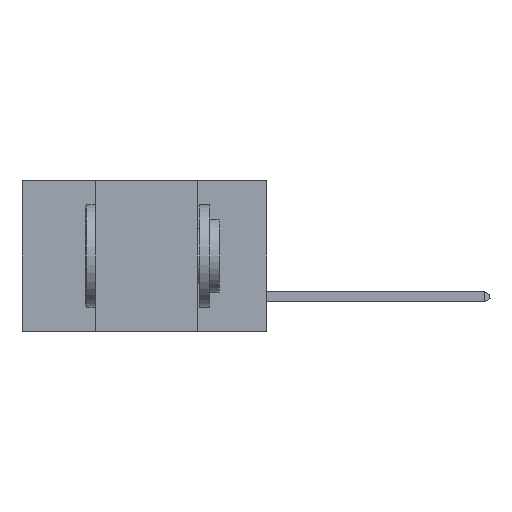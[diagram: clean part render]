
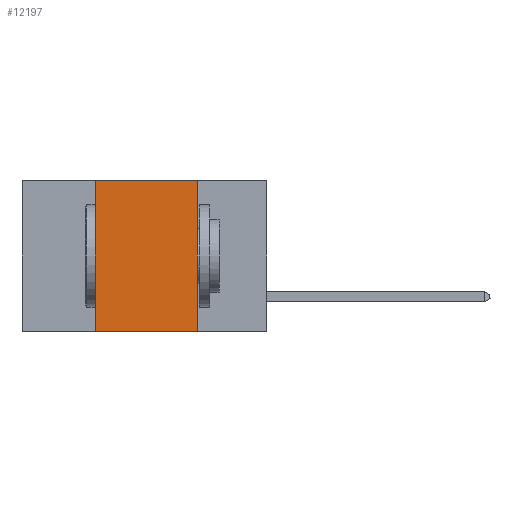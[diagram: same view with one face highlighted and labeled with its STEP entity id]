
A CAD part, left-side view. The second image highlights one B-rep face of the part: STEP entity #12197.
In plain terms, the highlighted planar face has unit normal (-1, 0, 0).
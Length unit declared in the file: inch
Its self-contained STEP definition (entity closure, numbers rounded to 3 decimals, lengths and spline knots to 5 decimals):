
#251 = VERTEX_POINT ( 'NONE', #5278 ) ;
#381 = ORIENTED_EDGE ( 'NONE', *, *, #16866, .F. ) ;
#1096 = CARTESIAN_POINT ( 'NONE',  ( 0., 0.6, 0. ) ) ;
#2161 = VECTOR ( 'NONE', #2471, 39.37008 ) ;
#2237 = VERTEX_POINT ( 'NONE', #14356 ) ;
#2471 = DIRECTION ( 'NONE',  ( 0., 0., -1. ) ) ;
#2515 = DIRECTION ( 'NONE',  ( 1., 0., 0. ) ) ;
#2875 = CARTESIAN_POINT ( 'NONE',  ( 0., 0.17, -0.37 ) ) ;
#2968 = DIRECTION ( 'NONE',  ( 0., 0., 1. ) ) ;
#5221 = DIRECTION ( 'NONE',  ( 0., -1., 0. ) ) ;
#5278 = CARTESIAN_POINT ( 'NONE',  ( 0., 0.42, 0. ) ) ;
#6181 = CARTESIAN_POINT ( 'NONE',  ( 0., 0.6, -0.37 ) ) ;
#6931 = LINE ( 'NONE', #6181, #9539 ) ;
#7085 = EDGE_CURVE ( 'NONE', #251, #2237, #10203, .T. ) ;
#7396 = DIRECTION ( 'NONE',  ( 0., -1., 0. ) ) ;
#8160 = VERTEX_POINT ( 'NONE', #2875 ) ;
#8296 = LINE ( 'NONE', #12520, #2161 ) ;
#8440 = CARTESIAN_POINT ( 'NONE',  ( 0., 0.42, 0. ) ) ;
#8703 = LINE ( 'NONE', #8440, #13141 ) ;
#9539 = VECTOR ( 'NONE', #7396, 39.37008 ) ;
#9577 = EDGE_CURVE ( 'NONE', #2237, #8160, #8296, .T. ) ;
#10203 = LINE ( 'NONE', #13533, #14189 ) ;
#10570 = EDGE_LOOP ( 'NONE', ( #16639, #10854, #381, #11951 ) ) ;
#10854 = ORIENTED_EDGE ( 'NONE', *, *, #7085, .F. ) ;
#11951 = ORIENTED_EDGE ( 'NONE', *, *, #14147, .T. ) ;
#12197 = ADVANCED_FACE ( 'NONE', ( #12381 ), #18047, .F. ) ;
#12381 = FACE_OUTER_BOUND ( 'NONE', #10570, .T. ) ;
#12520 = CARTESIAN_POINT ( 'NONE',  ( 0., 0.17, 0. ) ) ;
#12607 = CARTESIAN_POINT ( 'NONE',  ( 0., 0.42, -0.37 ) ) ;
#13141 = VECTOR ( 'NONE', #2968, 39.37008 ) ;
#13271 = AXIS2_PLACEMENT_3D ( 'NONE', #1096, #2515, #16726 ) ;
#13533 = CARTESIAN_POINT ( 'NONE',  ( 0., 0.6, 0. ) ) ;
#13577 = VERTEX_POINT ( 'NONE', #12607 ) ;
#14147 = EDGE_CURVE ( 'NONE', #13577, #8160, #6931, .T. ) ;
#14189 = VECTOR ( 'NONE', #5221, 39.37008 ) ;
#14356 = CARTESIAN_POINT ( 'NONE',  ( 0., 0.17, 0. ) ) ;
#16639 = ORIENTED_EDGE ( 'NONE', *, *, #9577, .F. ) ;
#16726 = DIRECTION ( 'NONE',  ( 0., 0., -1. ) ) ;
#16866 = EDGE_CURVE ( 'NONE', #13577, #251, #8703, .T. ) ;
#18047 = PLANE ( 'NONE',  #13271 ) ;
